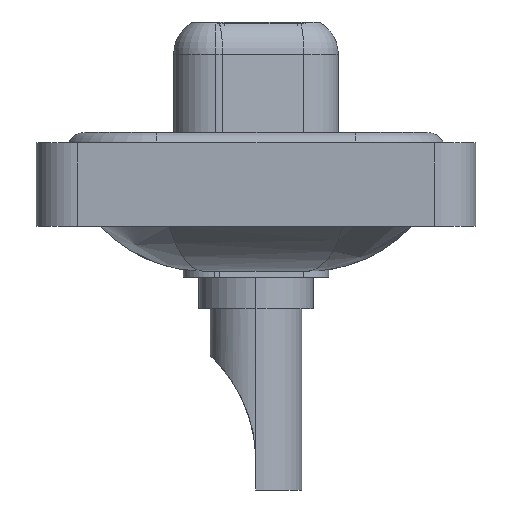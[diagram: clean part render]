
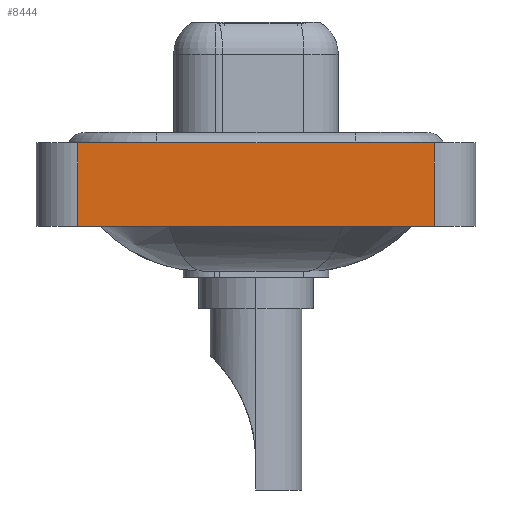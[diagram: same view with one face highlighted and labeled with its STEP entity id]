
A CAD part, left-side view. The second image highlights one B-rep face of the part: STEP entity #8444.
In plain terms, the highlighted planar face has unit normal (-1, 0, 0).
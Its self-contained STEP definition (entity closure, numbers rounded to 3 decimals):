
#223 = EDGE_CURVE ( 'NONE', #7019, #6363, #15598, .T. ) ;
#780 = CARTESIAN_POINT ( 'NONE',  ( -7.3, -8.55, 0.4 ) ) ;
#936 = ORIENTED_EDGE ( 'NONE', *, *, #14708, .T. ) ;
#1172 = EDGE_LOOP ( 'NONE', ( #936, #3279, #12145, #13946 ) ) ;
#1252 = VECTOR ( 'NONE', #8684, 1000. ) ;
#1934 = AXIS2_PLACEMENT_3D ( 'NONE', #6847, #12220, #4116 ) ;
#1935 = CARTESIAN_POINT ( 'NONE',  ( -7.3, -8.55, -3.6 ) ) ;
#3133 = CARTESIAN_POINT ( 'NONE',  ( -7.3, 8.55, -3.6 ) ) ;
#3279 = ORIENTED_EDGE ( 'NONE', *, *, #17437, .F. ) ;
#3481 = LINE ( 'NONE', #780, #7818 ) ;
#4116 = DIRECTION ( 'NONE',  ( 0., 0., 1. ) ) ;
#4204 = PLANE ( 'NONE',  #1934 ) ;
#5021 = CARTESIAN_POINT ( 'NONE',  ( -7.3, 8.55, -3.6 ) ) ;
#6363 = VERTEX_POINT ( 'NONE', #11352 ) ;
#6402 = DIRECTION ( 'NONE',  ( 0., -1., 0. ) ) ;
#6528 = VECTOR ( 'NONE', #15762, 1000. ) ;
#6643 = VECTOR ( 'NONE', #13467, 1000. ) ;
#6847 = CARTESIAN_POINT ( 'NONE',  ( -7.3, -8.55, -3.6 ) ) ;
#7019 = VERTEX_POINT ( 'NONE', #5021 ) ;
#7021 = CARTESIAN_POINT ( 'NONE',  ( -7.3, -8.55, -3.6 ) ) ;
#7205 = LINE ( 'NONE', #1935, #6528 ) ;
#7818 = VECTOR ( 'NONE', #6402, 1000. ) ;
#8444 = ADVANCED_FACE ( 'NONE', ( #9399 ), #4204, .T. ) ;
#8684 = DIRECTION ( 'NONE',  ( 0., 0., 1. ) ) ;
#9078 = VERTEX_POINT ( 'NONE', #16542 ) ;
#9399 = FACE_OUTER_BOUND ( 'NONE', #1172, .T. ) ;
#11053 = EDGE_CURVE ( 'NONE', #7019, #17269, #13738, .T. ) ;
#11352 = CARTESIAN_POINT ( 'NONE',  ( -7.3, 8.55, 0.4 ) ) ;
#12145 = ORIENTED_EDGE ( 'NONE', *, *, #223, .F. ) ;
#12220 = DIRECTION ( 'NONE',  ( -1., 0., 0. ) ) ;
#13467 = DIRECTION ( 'NONE',  ( 0., -1., 0. ) ) ;
#13738 = LINE ( 'NONE', #15017, #6643 ) ;
#13946 = ORIENTED_EDGE ( 'NONE', *, *, #11053, .T. ) ;
#14708 = EDGE_CURVE ( 'NONE', #17269, #9078, #7205, .T. ) ;
#15017 = CARTESIAN_POINT ( 'NONE',  ( -7.3, -8.55, -3.6 ) ) ;
#15598 = LINE ( 'NONE', #3133, #1252 ) ;
#15762 = DIRECTION ( 'NONE',  ( 0., 0., 1. ) ) ;
#16542 = CARTESIAN_POINT ( 'NONE',  ( -7.3, -8.55, 0.4 ) ) ;
#17269 = VERTEX_POINT ( 'NONE', #7021 ) ;
#17437 = EDGE_CURVE ( 'NONE', #6363, #9078, #3481, .T. ) ;
